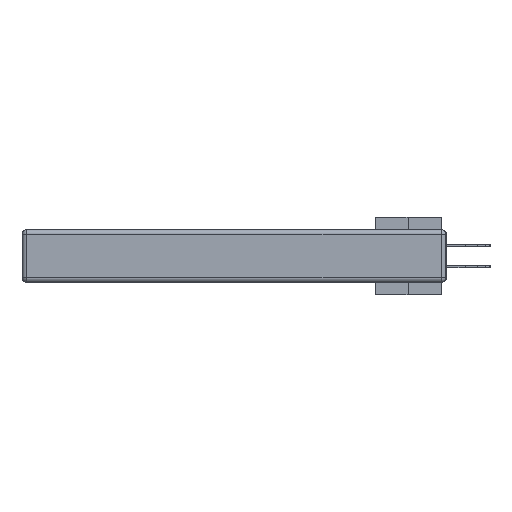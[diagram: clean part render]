
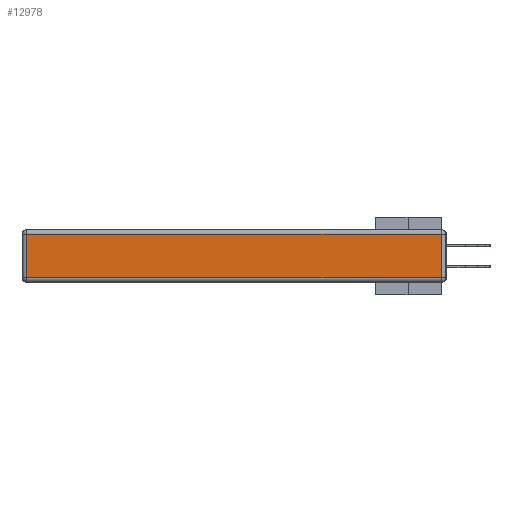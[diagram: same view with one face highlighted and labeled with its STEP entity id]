
A CAD part, left-side view. The second image highlights one B-rep face of the part: STEP entity #12978.
In plain terms, the highlighted planar face has unit normal (-1, 0, 0).
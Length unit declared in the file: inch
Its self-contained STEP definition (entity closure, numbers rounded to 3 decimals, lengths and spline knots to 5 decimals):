
#287 = CARTESIAN_POINT ( 'NONE',  ( 0., 2.72, -0.03 ) ) ;
#2045 = VECTOR ( 'NONE', #3528, 39.37008 ) ;
#2509 = VERTEX_POINT ( 'NONE', #38922 ) ;
#2986 = ORIENTED_EDGE ( 'NONE', *, *, #43164, .T. ) ;
#3139 = CARTESIAN_POINT ( 'NONE',  ( 0., 0.03, -0.03 ) ) ;
#3528 = DIRECTION ( 'NONE',  ( 0., 0., 1. ) ) ;
#5784 = VECTOR ( 'NONE', #32731, 39.37008 ) ;
#6097 = VERTEX_POINT ( 'NONE', #287 ) ;
#7727 = DIRECTION ( 'NONE',  ( -1., 0., 0. ) ) ;
#7820 = CARTESIAN_POINT ( 'NONE',  ( 0., 0., -0.313 ) ) ;
#8994 = VERTEX_POINT ( 'NONE', #3139 ) ;
#9024 = ORIENTED_EDGE ( 'NONE', *, *, #36714, .T. ) ;
#9059 = DIRECTION ( 'NONE',  ( 0., -1., 0. ) ) ;
#11003 = DIRECTION ( 'NONE',  ( 0., 0., -1. ) ) ;
#12978 = ADVANCED_FACE ( 'NONE', ( #31788 ), #36178, .T. ) ;
#17417 = EDGE_CURVE ( 'NONE', #2509, #8994, #44333, .T. ) ;
#18027 = CARTESIAN_POINT ( 'NONE',  ( 0., 0.03, -0.343 ) ) ;
#20112 = EDGE_LOOP ( 'NONE', ( #9024, #26264, #30507, #2986 ) ) ;
#20580 = VECTOR ( 'NONE', #9059, 39.37008 ) ;
#21719 = EDGE_CURVE ( 'NONE', #8994, #6097, #24663, .T. ) ;
#24663 = LINE ( 'NONE', #40251, #5784 ) ;
#24988 = VECTOR ( 'NONE', #11003, 39.37008 ) ;
#25529 = DIRECTION ( 'NONE',  ( 0., 0., 1. ) ) ;
#26264 = ORIENTED_EDGE ( 'NONE', *, *, #17417, .T. ) ;
#29143 = CARTESIAN_POINT ( 'NONE',  ( 0., 2.72, -0.343 ) ) ;
#30308 = LINE ( 'NONE', #7820, #20580 ) ;
#30507 = ORIENTED_EDGE ( 'NONE', *, *, #21719, .T. ) ;
#31736 = CARTESIAN_POINT ( 'NONE',  ( 0., 2.72, -0.313 ) ) ;
#31788 = FACE_OUTER_BOUND ( 'NONE', #20112, .T. ) ;
#32525 = VERTEX_POINT ( 'NONE', #31736 ) ;
#32668 = CARTESIAN_POINT ( 'NONE',  ( 0., 0., -0.343 ) ) ;
#32731 = DIRECTION ( 'NONE',  ( 0., 1., 0. ) ) ;
#34702 = AXIS2_PLACEMENT_3D ( 'NONE', #32668, #7727, #25529 ) ;
#36178 = PLANE ( 'NONE',  #34702 ) ;
#36714 = EDGE_CURVE ( 'NONE', #32525, #2509, #30308, .T. ) ;
#38922 = CARTESIAN_POINT ( 'NONE',  ( 0., 0.03, -0.313 ) ) ;
#40251 = CARTESIAN_POINT ( 'NONE',  ( 0., 2.75, -0.03 ) ) ;
#41559 = LINE ( 'NONE', #29143, #24988 ) ;
#43164 = EDGE_CURVE ( 'NONE', #6097, #32525, #41559, .T. ) ;
#44333 = LINE ( 'NONE', #18027, #2045 ) ;
